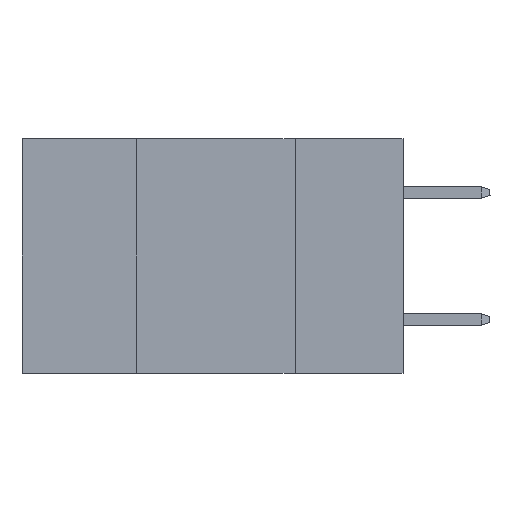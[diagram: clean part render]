
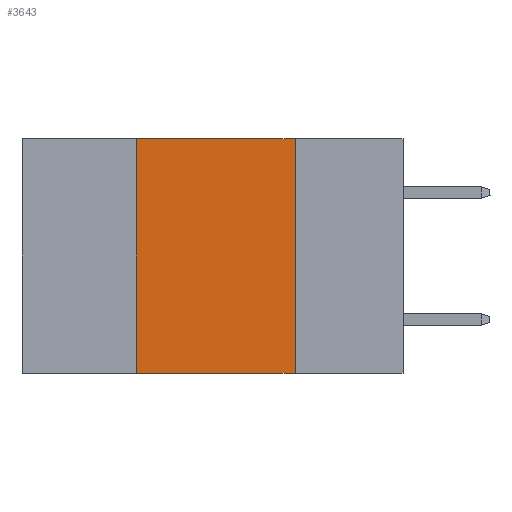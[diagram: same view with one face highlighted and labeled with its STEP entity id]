
A CAD part, left-side view. The second image highlights one B-rep face of the part: STEP entity #3643.
In plain terms, the highlighted planar face has unit normal (-1, 0, 0).
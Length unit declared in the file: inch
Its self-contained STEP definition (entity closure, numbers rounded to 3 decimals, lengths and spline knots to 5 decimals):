
#118 = EDGE_CURVE ( 'NONE', #9259, #7290, #7115, .T. ) ;
#303 = VECTOR ( 'NONE', #10589, 39.37008 ) ;
#436 = ORIENTED_EDGE ( 'NONE', *, *, #7083, .F. ) ;
#474 = ORIENTED_EDGE ( 'NONE', *, *, #118, .F. ) ;
#1266 = VERTEX_POINT ( 'NONE', #2036 ) ;
#1376 = AXIS2_PLACEMENT_3D ( 'NONE', #5416, #6275, #7846 ) ;
#1872 = FACE_OUTER_BOUND ( 'NONE', #9477, .T. ) ;
#2036 = CARTESIAN_POINT ( 'NONE',  ( 0., 0.42, -0.37 ) ) ;
#2735 = CARTESIAN_POINT ( 'NONE',  ( 0., 0.42, 0. ) ) ;
#2988 = ORIENTED_EDGE ( 'NONE', *, *, #8938, .F. ) ;
#3643 = ADVANCED_FACE ( 'NONE', ( #1872 ), #8667, .F. ) ;
#3751 = CARTESIAN_POINT ( 'NONE',  ( 0., 0.17, 0. ) ) ;
#3884 = LINE ( 'NONE', #8252, #8662 ) ;
#3953 = CARTESIAN_POINT ( 'NONE',  ( 0., 0.6, 0. ) ) ;
#4871 = CARTESIAN_POINT ( 'NONE',  ( 0., 0.17, 0. ) ) ;
#4915 = VECTOR ( 'NONE', #5233, 39.37008 ) ;
#5233 = DIRECTION ( 'NONE',  ( 0., -1., 0. ) ) ;
#5416 = CARTESIAN_POINT ( 'NONE',  ( 0., 0.6, 0. ) ) ;
#5512 = LINE ( 'NONE', #5914, #4915 ) ;
#5914 = CARTESIAN_POINT ( 'NONE',  ( 0., 0.6, -0.37 ) ) ;
#6275 = DIRECTION ( 'NONE',  ( 1., 0., 0. ) ) ;
#6350 = VERTEX_POINT ( 'NONE', #2735 ) ;
#7083 = EDGE_CURVE ( 'NONE', #6350, #9259, #8992, .T. ) ;
#7115 = LINE ( 'NONE', #3751, #303 ) ;
#7253 = DIRECTION ( 'NONE',  ( 0., -1., 0. ) ) ;
#7290 = VERTEX_POINT ( 'NONE', #10125 ) ;
#7846 = DIRECTION ( 'NONE',  ( 0., 0., -1. ) ) ;
#8252 = CARTESIAN_POINT ( 'NONE',  ( 0., 0.42, 0. ) ) ;
#8662 = VECTOR ( 'NONE', #9935, 39.37008 ) ;
#8667 = PLANE ( 'NONE',  #1376 ) ;
#8938 = EDGE_CURVE ( 'NONE', #1266, #6350, #3884, .T. ) ;
#8992 = LINE ( 'NONE', #3953, #9497 ) ;
#9259 = VERTEX_POINT ( 'NONE', #4871 ) ;
#9477 = EDGE_LOOP ( 'NONE', ( #474, #436, #2988, #10213 ) ) ;
#9497 = VECTOR ( 'NONE', #7253, 39.37008 ) ;
#9542 = EDGE_CURVE ( 'NONE', #1266, #7290, #5512, .T. ) ;
#9935 = DIRECTION ( 'NONE',  ( 0., 0., 1. ) ) ;
#10125 = CARTESIAN_POINT ( 'NONE',  ( 0., 0.17, -0.37 ) ) ;
#10213 = ORIENTED_EDGE ( 'NONE', *, *, #9542, .T. ) ;
#10589 = DIRECTION ( 'NONE',  ( 0., 0., -1. ) ) ;
